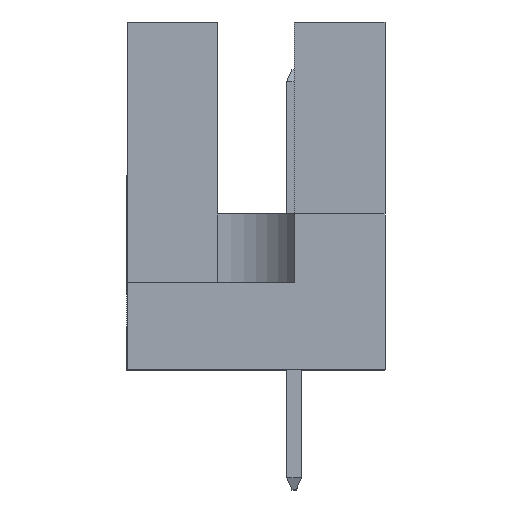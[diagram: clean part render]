
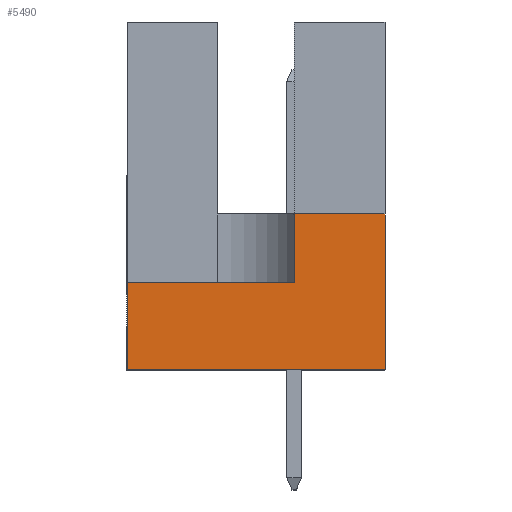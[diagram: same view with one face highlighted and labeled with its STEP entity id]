
A CAD part, left-side view. The second image highlights one B-rep face of the part: STEP entity #5490.
In plain terms, the highlighted planar face has unit normal (-1, 0, 0).
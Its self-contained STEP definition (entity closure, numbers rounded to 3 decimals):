
#637 = EDGE_CURVE ( 'NONE', #3362, #9560, #4164, .T. ) ;
#901 = CARTESIAN_POINT ( 'NONE',  ( -47.5, -1.27, 2.9 ) ) ;
#1077 = VERTEX_POINT ( 'NONE', #2231 ) ;
#1129 = VERTEX_POINT ( 'NONE', #901 ) ;
#1267 = EDGE_CURVE ( 'NONE', #1129, #1077, #10799, .T. ) ;
#1429 = VECTOR ( 'NONE', #6409, 1000. ) ;
#1636 = CARTESIAN_POINT ( 'NONE',  ( -47.5, 4.3, 11.6 ) ) ;
#1977 = ORIENTED_EDGE ( 'NONE', *, *, #1267, .T. ) ;
#2231 = CARTESIAN_POINT ( 'NONE',  ( -47.5, 4.3, 2.9 ) ) ;
#2300 = DIRECTION ( 'NONE',  ( 0., 0., -1. ) ) ;
#2306 = ORIENTED_EDGE ( 'NONE', *, *, #5559, .T. ) ;
#2368 = PLANE ( 'NONE',  #8069 ) ;
#2405 = VECTOR ( 'NONE', #4352, 1000. ) ;
#2561 = EDGE_CURVE ( 'NONE', #5784, #1129, #6237, .T. ) ;
#2593 = CARTESIAN_POINT ( 'NONE',  ( -47.5, 4.3, 2.9 ) ) ;
#2683 = CARTESIAN_POINT ( 'NONE',  ( -47.5, 4.3, 0. ) ) ;
#2722 = DIRECTION ( 'NONE',  ( 0., 0., -1. ) ) ;
#2994 = VECTOR ( 'NONE', #10362, 1000. ) ;
#3140 = EDGE_LOOP ( 'NONE', ( #10158, #9783, #1977, #2306, #5661, #3677 ) ) ;
#3227 = CARTESIAN_POINT ( 'NONE',  ( -47.5, -1.27, 5.2 ) ) ;
#3362 = VERTEX_POINT ( 'NONE', #9562 ) ;
#3377 = CARTESIAN_POINT ( 'NONE',  ( -47.5, -4.3, 11.6 ) ) ;
#3442 = CARTESIAN_POINT ( 'NONE',  ( -47.5, -4.3, 0. ) ) ;
#3665 = CARTESIAN_POINT ( 'NONE',  ( -47.5, -1.27, 19.02 ) ) ;
#3677 = ORIENTED_EDGE ( 'NONE', *, *, #637, .F. ) ;
#4164 = LINE ( 'NONE', #3377, #2405 ) ;
#4352 = DIRECTION ( 'NONE',  ( 0., 0., -1. ) ) ;
#5490 = ADVANCED_FACE ( 'NONE', ( #6847 ), #2368, .F. ) ;
#5559 = EDGE_CURVE ( 'NONE', #1077, #10373, #7337, .T. ) ;
#5661 = ORIENTED_EDGE ( 'NONE', *, *, #10034, .T. ) ;
#5744 = CARTESIAN_POINT ( 'NONE',  ( -47.5, 4.3, 5.2 ) ) ;
#5784 = VERTEX_POINT ( 'NONE', #3227 ) ;
#6237 = LINE ( 'NONE', #3665, #10957 ) ;
#6297 = DIRECTION ( 'NONE',  ( 0., 0., -1. ) ) ;
#6409 = DIRECTION ( 'NONE',  ( 0., 1., 0. ) ) ;
#6475 = CARTESIAN_POINT ( 'NONE',  ( -47.5, 4.3, 0. ) ) ;
#6847 = FACE_OUTER_BOUND ( 'NONE', #3140, .T. ) ;
#7337 = LINE ( 'NONE', #1636, #10953 ) ;
#8069 = AXIS2_PLACEMENT_3D ( 'NONE', #9665, #10510, #2300 ) ;
#8224 = LINE ( 'NONE', #6475, #9686 ) ;
#9560 = VERTEX_POINT ( 'NONE', #3442 ) ;
#9562 = CARTESIAN_POINT ( 'NONE',  ( -47.5, -4.3, 5.2 ) ) ;
#9665 = CARTESIAN_POINT ( 'NONE',  ( -47.5, 4.3, 11.6 ) ) ;
#9686 = VECTOR ( 'NONE', #10345, 1000. ) ;
#9783 = ORIENTED_EDGE ( 'NONE', *, *, #2561, .T. ) ;
#10034 = EDGE_CURVE ( 'NONE', #10373, #9560, #8224, .T. ) ;
#10158 = ORIENTED_EDGE ( 'NONE', *, *, #11568, .F. ) ;
#10345 = DIRECTION ( 'NONE',  ( 0., -1., 0. ) ) ;
#10362 = DIRECTION ( 'NONE',  ( 0., -1., 0. ) ) ;
#10373 = VERTEX_POINT ( 'NONE', #2683 ) ;
#10421 = LINE ( 'NONE', #5744, #2994 ) ;
#10510 = DIRECTION ( 'NONE',  ( 1., 0., 0. ) ) ;
#10799 = LINE ( 'NONE', #2593, #1429 ) ;
#10953 = VECTOR ( 'NONE', #2722, 1000. ) ;
#10957 = VECTOR ( 'NONE', #6297, 1000. ) ;
#11568 = EDGE_CURVE ( 'NONE', #5784, #3362, #10421, .T. ) ;
